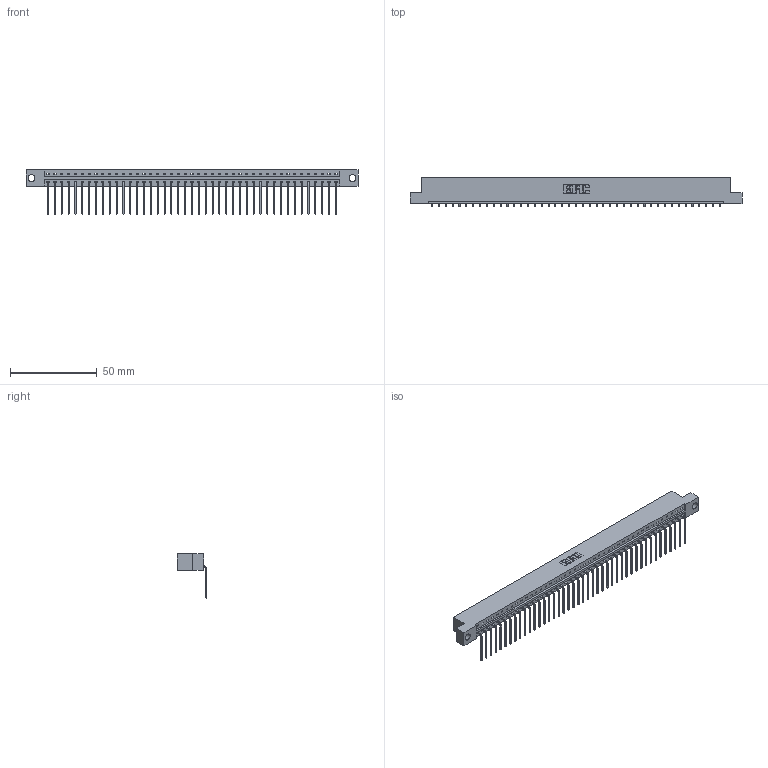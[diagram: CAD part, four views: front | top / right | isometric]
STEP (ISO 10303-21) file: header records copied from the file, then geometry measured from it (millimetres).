
FILE_DESCRIPTION (( 'STEP AP203' ), '1' );
FILE_NAME ('333-043-559-104.STEP', '2018-08-03T20:44:10', ( '' ), ( '' ), 'SwSTEP 2.0', 'SolidWorks 2016', '' );
FILE_SCHEMA (( 'CONFIG_CONTROL_DESIGN' ));
Length unit declared in the file: inch
Products named in the file (3): 333 Part_Flush - .156 Dia - TH; 345-292-001_558 559 Tail - 1; 333-043-559-104
Assembly tree (44 placements, depth 2):
  333-043-559-104
    333 Part_Flush - .156 Dia - TH
    345-292-001_558 559 Tail - 1  x43
Bounding box: 191.92 x 17.09 x 25.53 mm (x, y, z)
Volume: 19376.8 mm3; surface area: 21645.9 mm2
Topology: 44 solids, 44 shells, 2694 faces, 8137 edges, 5366 vertices
Faces by surface type: plane 1962, cylinder 732
Entity records: 26245 total; most frequent: CARTESIAN_POINT 4535, ORIENTED_EDGE 4514, DIRECTION 3823, EDGE_CURVE 2257, LINE 2129, VECTOR 2129, VERTEX_POINT 1502, AXIS2_PLACEMENT_3D 847
